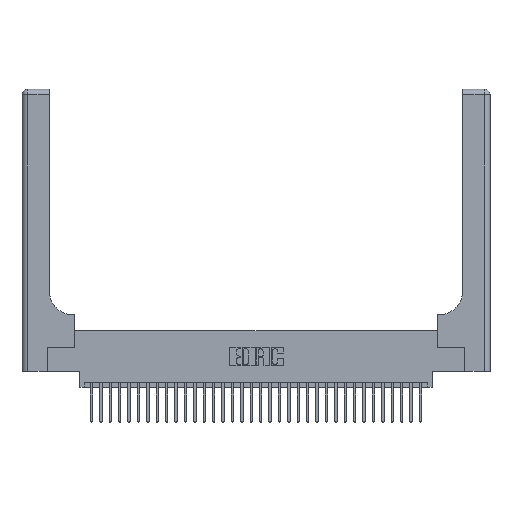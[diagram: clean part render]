
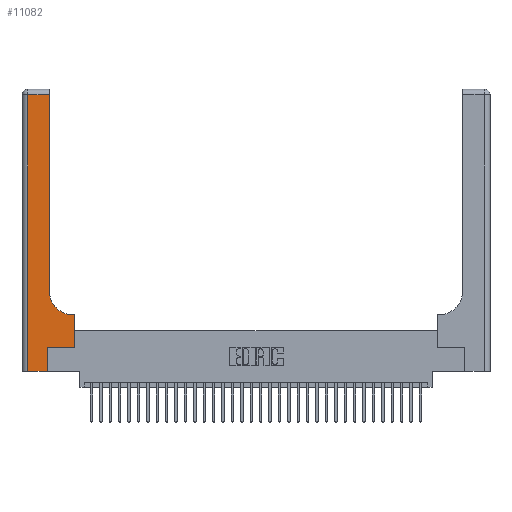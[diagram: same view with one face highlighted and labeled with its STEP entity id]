
A CAD part, top view. The second image highlights one B-rep face of the part: STEP entity #11082.
In plain terms, the highlighted planar face has unit normal (0, 0, 1).
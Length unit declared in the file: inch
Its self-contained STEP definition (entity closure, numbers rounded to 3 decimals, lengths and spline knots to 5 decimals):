
#2052 = VECTOR ( 'NONE', #7680, 39.37008 ) ;
#2297 = ORIENTED_EDGE ( 'NONE', *, *, #22615, .T. ) ;
#2324 = EDGE_CURVE ( 'NONE', #32406, #10526, #16790, .T. ) ;
#2571 = VECTOR ( 'NONE', #16141, 39.37008 ) ;
#3182 = CARTESIAN_POINT ( 'NONE',  ( 0.2915, 3., 0.37 ) ) ;
#3971 = VERTEX_POINT ( 'NONE', #4013 ) ;
#4013 = CARTESIAN_POINT ( 'NONE',  ( 0.06, 0., 0.37 ) ) ;
#4465 = LINE ( 'NONE', #24813, #31857 ) ;
#4508 = DIRECTION ( 'NONE',  ( 0., 0., -1. ) ) ;
#4779 = CARTESIAN_POINT ( 'NONE',  ( 0.5415, 0.85, 0.37 ) ) ;
#5344 = VERTEX_POINT ( 'NONE', #15016 ) ;
#6473 = CARTESIAN_POINT ( 'NONE',  ( 0.2915, 0.85, 0.37 ) ) ;
#7022 = CARTESIAN_POINT ( 'NONE',  ( 0., 0., 0.37 ) ) ;
#7457 = DIRECTION ( 'NONE',  ( 1., 0., 0. ) ) ;
#7680 = DIRECTION ( 'NONE',  ( 0., 1., 0. ) ) ;
#7796 = CARTESIAN_POINT ( 'NONE',  ( 0.5415, 0.6, 0.37 ) ) ;
#8076 = LINE ( 'NONE', #11525, #29256 ) ;
#8397 = CARTESIAN_POINT ( 'NONE',  ( 0.2915, 2.94, 0.37 ) ) ;
#8492 = AXIS2_PLACEMENT_3D ( 'NONE', #4779, #23374, #7457 ) ;
#9209 = LINE ( 'NONE', #31423, #2052 ) ;
#9749 = DIRECTION ( 'NONE',  ( 1., 0., 0. ) ) ;
#9999 = AXIS2_PLACEMENT_3D ( 'NONE', #20495, #4508, #23136 ) ;
#10526 = VERTEX_POINT ( 'NONE', #7796 ) ;
#10537 = ORIENTED_EDGE ( 'NONE', *, *, #29231, .T. ) ;
#10905 = CARTESIAN_POINT ( 'NONE',  ( 0., 2.94, 0.37 ) ) ;
#11049 = VERTEX_POINT ( 'NONE', #20362 ) ;
#11082 = ADVANCED_FACE ( 'NONE', ( #11945 ), #17813, .F. ) ;
#11525 = CARTESIAN_POINT ( 'NONE',  ( 0.269, 0., 0.37 ) ) ;
#11945 = FACE_OUTER_BOUND ( 'NONE', #33499, .T. ) ;
#12541 = EDGE_CURVE ( 'NONE', #17533, #11049, #21809, .T. ) ;
#13112 = EDGE_CURVE ( 'NONE', #21991, #29741, #14370, .T. ) ;
#13387 = VERTEX_POINT ( 'NONE', #6473 ) ;
#13489 = CARTESIAN_POINT ( 'NONE',  ( 0.2915, 0.6, 0.37 ) ) ;
#13980 = DIRECTION ( 'NONE',  ( 0., 1., 0. ) ) ;
#14081 = CIRCLE ( 'NONE', #8492, 0.25 ) ;
#14370 = LINE ( 'NONE', #23826, #20572 ) ;
#14535 = VECTOR ( 'NONE', #9749, 39.37008 ) ;
#14753 = VECTOR ( 'NONE', #21578, 39.37008 ) ;
#15016 = CARTESIAN_POINT ( 'NONE',  ( 0.269, 0., 0.37 ) ) ;
#15352 = LINE ( 'NONE', #7022, #14535 ) ;
#16141 = DIRECTION ( 'NONE',  ( -1., 0., 0. ) ) ;
#16713 = ORIENTED_EDGE ( 'NONE', *, *, #12541, .T. ) ;
#16790 = LINE ( 'NONE', #13489, #2571 ) ;
#17533 = VERTEX_POINT ( 'NONE', #8397 ) ;
#17813 = PLANE ( 'NONE',  #9999 ) ;
#19093 = CARTESIAN_POINT ( 'NONE',  ( 0.269, 0.25, 0.37 ) ) ;
#19935 = ORIENTED_EDGE ( 'NONE', *, *, #34237, .T. ) ;
#20362 = CARTESIAN_POINT ( 'NONE',  ( 0.06, 2.94, 0.37 ) ) ;
#20495 = CARTESIAN_POINT ( 'NONE',  ( 0., 3., 0.37 ) ) ;
#20572 = VECTOR ( 'NONE', #31534, 39.37008 ) ;
#21578 = DIRECTION ( 'NONE',  ( -1., 0., 0. ) ) ;
#21809 = LINE ( 'NONE', #10905, #14753 ) ;
#21991 = VERTEX_POINT ( 'NONE', #19093 ) ;
#22145 = EDGE_CURVE ( 'NONE', #11049, #3971, #4465, .T. ) ;
#22615 = EDGE_CURVE ( 'NONE', #13387, #17533, #25635, .T. ) ;
#23136 = DIRECTION ( 'NONE',  ( -1., 0., 0. ) ) ;
#23374 = DIRECTION ( 'NONE',  ( 0., 0., -1. ) ) ;
#23826 = CARTESIAN_POINT ( 'NONE',  ( 0.269, 0.25, 0.37 ) ) ;
#24536 = EDGE_CURVE ( 'NONE', #5344, #21991, #8076, .T. ) ;
#24559 = ORIENTED_EDGE ( 'NONE', *, *, #22145, .T. ) ;
#24810 = VECTOR ( 'NONE', #13980, 39.37008 ) ;
#24813 = CARTESIAN_POINT ( 'NONE',  ( 0.06, 3., 0.37 ) ) ;
#25635 = LINE ( 'NONE', #3182, #24810 ) ;
#25747 = ORIENTED_EDGE ( 'NONE', *, *, #29913, .T. ) ;
#27553 = CARTESIAN_POINT ( 'NONE',  ( 0.5585, 0.25, 0.37 ) ) ;
#28898 = CARTESIAN_POINT ( 'NONE',  ( 0.5585, 0.6, 0.37 ) ) ;
#29231 = EDGE_CURVE ( 'NONE', #3971, #5344, #15352, .T. ) ;
#29256 = VECTOR ( 'NONE', #30005, 39.37008 ) ;
#29741 = VERTEX_POINT ( 'NONE', #27553 ) ;
#29913 = EDGE_CURVE ( 'NONE', #10526, #13387, #14081, .T. ) ;
#30005 = DIRECTION ( 'NONE',  ( 0., 1., 0. ) ) ;
#30139 = DIRECTION ( 'NONE',  ( 0., -1., 0. ) ) ;
#30591 = ORIENTED_EDGE ( 'NONE', *, *, #24536, .T. ) ;
#31423 = CARTESIAN_POINT ( 'NONE',  ( 0.5585, 0.25, 0.37 ) ) ;
#31534 = DIRECTION ( 'NONE',  ( 1., 0., 0. ) ) ;
#31857 = VECTOR ( 'NONE', #30139, 39.37008 ) ;
#32406 = VERTEX_POINT ( 'NONE', #28898 ) ;
#32592 = ORIENTED_EDGE ( 'NONE', *, *, #13112, .T. ) ;
#33207 = ORIENTED_EDGE ( 'NONE', *, *, #2324, .T. ) ;
#33499 = EDGE_LOOP ( 'NONE', ( #2297, #16713, #24559, #10537, #30591, #32592, #19935, #33207, #25747 ) ) ;
#34237 = EDGE_CURVE ( 'NONE', #29741, #32406, #9209, .T. ) ;
